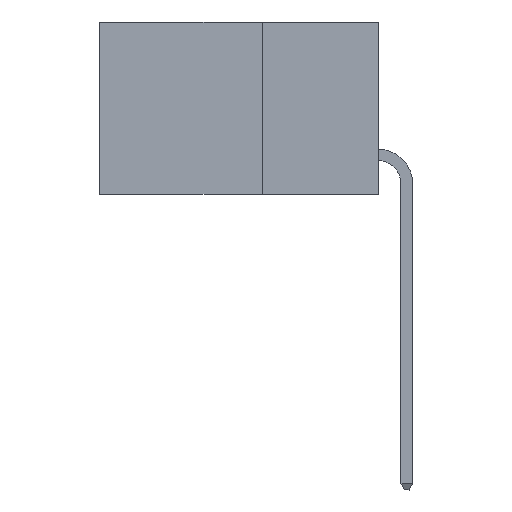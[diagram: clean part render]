
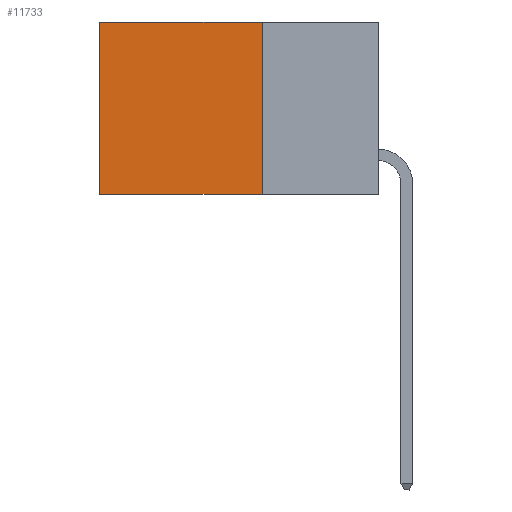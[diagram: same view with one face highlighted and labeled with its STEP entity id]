
A CAD part, left-side view. The second image highlights one B-rep face of the part: STEP entity #11733.
In plain terms, the highlighted planar face has unit normal (-1, 0, 0).
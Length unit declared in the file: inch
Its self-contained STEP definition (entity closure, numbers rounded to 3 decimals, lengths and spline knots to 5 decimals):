
#58 = EDGE_CURVE ( 'NONE', #15969, #12314, #8237, .T. ) ;
#1371 = EDGE_LOOP ( 'NONE', ( #2319, #2243, #2166, #2153 ) ) ;
#1833 = DIRECTION ( 'NONE',  ( 0., 1., 0. ) ) ;
#1854 = CARTESIAN_POINT ( 'NONE',  ( 0.298, 0.25, -0.37 ) ) ;
#2153 = ORIENTED_EDGE ( 'NONE', *, *, #8649, .T. ) ;
#2166 = ORIENTED_EDGE ( 'NONE', *, *, #5453, .F. ) ;
#2243 = ORIENTED_EDGE ( 'NONE', *, *, #58, .F. ) ;
#2319 = ORIENTED_EDGE ( 'NONE', *, *, #10654, .T. ) ;
#2686 = DIRECTION ( 'NONE',  ( 1., 0., 0. ) ) ;
#3921 = VECTOR ( 'NONE', #10345, 39.37008 ) ;
#4239 = VERTEX_POINT ( 'NONE', #11523 ) ;
#4711 = DIRECTION ( 'NONE',  ( 0., 1., 0. ) ) ;
#4793 = CARTESIAN_POINT ( 'NONE',  ( 0.298, 0.25, 0. ) ) ;
#5096 = DIRECTION ( 'NONE',  ( 0., 0., -1. ) ) ;
#5259 = VECTOR ( 'NONE', #1833, 39.37008 ) ;
#5447 = VECTOR ( 'NONE', #4711, 39.37008 ) ;
#5453 = EDGE_CURVE ( 'NONE', #4239, #15969, #13227, .T. ) ;
#5735 = CARTESIAN_POINT ( 'NONE',  ( 0.298, 0.25, -0.37 ) ) ;
#7337 = LINE ( 'NONE', #12779, #3921 ) ;
#7807 = CARTESIAN_POINT ( 'NONE',  ( 0.298, 0.6, 0. ) ) ;
#8237 = LINE ( 'NONE', #1854, #5259 ) ;
#8649 = EDGE_CURVE ( 'NONE', #4239, #11746, #15191, .T. ) ;
#9008 = CARTESIAN_POINT ( 'NONE',  ( 0.298, 0.25, 0. ) ) ;
#9052 = FACE_OUTER_BOUND ( 'NONE', #1371, .T. ) ;
#10345 = DIRECTION ( 'NONE',  ( 0., 0., -1. ) ) ;
#10654 = EDGE_CURVE ( 'NONE', #11746, #12314, #7337, .T. ) ;
#11356 = PLANE ( 'NONE',  #11453 ) ;
#11408 = DIRECTION ( 'NONE',  ( 0., 0., -1. ) ) ;
#11453 = AXIS2_PLACEMENT_3D ( 'NONE', #9008, #2686, #11408 ) ;
#11523 = CARTESIAN_POINT ( 'NONE',  ( 0.298, 0.25, 0. ) ) ;
#11733 = ADVANCED_FACE ( 'NONE', ( #9052 ), #11356, .F. ) ;
#11746 = VERTEX_POINT ( 'NONE', #7807 ) ;
#12314 = VERTEX_POINT ( 'NONE', #12506 ) ;
#12506 = CARTESIAN_POINT ( 'NONE',  ( 0.298, 0.6, -0.37 ) ) ;
#12779 = CARTESIAN_POINT ( 'NONE',  ( 0.298, 0.6, 0. ) ) ;
#13227 = LINE ( 'NONE', #4793, #15664 ) ;
#15191 = LINE ( 'NONE', #15727, #5447 ) ;
#15664 = VECTOR ( 'NONE', #5096, 39.37008 ) ;
#15727 = CARTESIAN_POINT ( 'NONE',  ( 0.298, 0.25, 0. ) ) ;
#15969 = VERTEX_POINT ( 'NONE', #5735 ) ;
